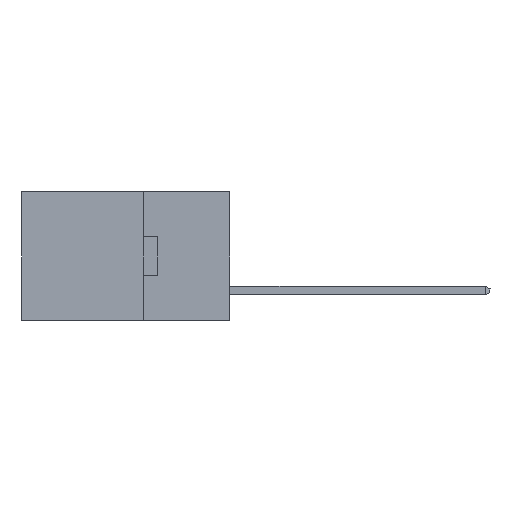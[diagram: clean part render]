
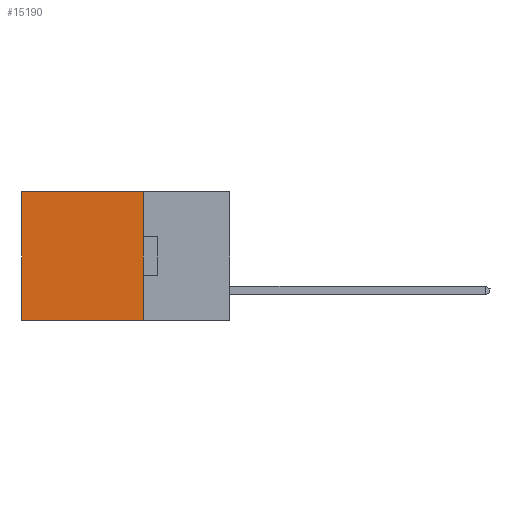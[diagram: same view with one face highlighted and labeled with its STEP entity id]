
A CAD part, left-side view. The second image highlights one B-rep face of the part: STEP entity #15190.
In plain terms, the highlighted planar face has unit normal (-1, 0, 0).
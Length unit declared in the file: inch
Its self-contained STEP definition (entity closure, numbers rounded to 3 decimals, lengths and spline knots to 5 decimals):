
#1977 = DIRECTION ( 'NONE',  ( 0., 1., 0. ) ) ;
#2540 = CARTESIAN_POINT ( 'NONE',  ( 0.2615, 0.6, -0.37 ) ) ;
#4288 = EDGE_LOOP ( 'NONE', ( #26540, #19473, #7708, #11205 ) ) ;
#7142 = VERTEX_POINT ( 'NONE', #14730 ) ;
#7708 = ORIENTED_EDGE ( 'NONE', *, *, #24120, .F. ) ;
#8115 = CARTESIAN_POINT ( 'NONE',  ( 0.2615, 0.25, -0.37 ) ) ;
#9136 = LINE ( 'NONE', #2540, #27112 ) ;
#9703 = DIRECTION ( 'NONE',  ( 0., 0., -1. ) ) ;
#11191 = VECTOR ( 'NONE', #24439, 39.37008 ) ;
#11205 = ORIENTED_EDGE ( 'NONE', *, *, #12242, .T. ) ;
#12172 = CARTESIAN_POINT ( 'NONE',  ( 0.2615, 0.25, 0. ) ) ;
#12242 = EDGE_CURVE ( 'NONE', #23742, #7142, #24299, .T. ) ;
#13136 = CARTESIAN_POINT ( 'NONE',  ( 0.2615, 0.6, -0.37 ) ) ;
#14111 = EDGE_CURVE ( 'NONE', #15442, #15092, #14887, .T. ) ;
#14730 = CARTESIAN_POINT ( 'NONE',  ( 0.2615, 0.6, 0. ) ) ;
#14887 = LINE ( 'NONE', #27142, #22099 ) ;
#15020 = CARTESIAN_POINT ( 'NONE',  ( 0.2615, 0.25, -0.37 ) ) ;
#15092 = VERTEX_POINT ( 'NONE', #13136 ) ;
#15190 = ADVANCED_FACE ( 'NONE', ( #18088 ), #22358, .F. ) ;
#15442 = VERTEX_POINT ( 'NONE', #15020 ) ;
#16292 = CARTESIAN_POINT ( 'NONE',  ( 0.2615, 0.25, -0.37 ) ) ;
#18001 = VECTOR ( 'NONE', #23085, 39.37008 ) ;
#18088 = FACE_OUTER_BOUND ( 'NONE', #4288, .T. ) ;
#18872 = EDGE_CURVE ( 'NONE', #7142, #15092, #9136, .T. ) ;
#19466 = DIRECTION ( 'NONE',  ( 0., 0., -1. ) ) ;
#19473 = ORIENTED_EDGE ( 'NONE', *, *, #14111, .F. ) ;
#20189 = CARTESIAN_POINT ( 'NONE',  ( 0.2615, 0.25, 0. ) ) ;
#22099 = VECTOR ( 'NONE', #1977, 39.37008 ) ;
#22358 = PLANE ( 'NONE',  #26960 ) ;
#22691 = LINE ( 'NONE', #8115, #18001 ) ;
#23085 = DIRECTION ( 'NONE',  ( 0., 0., -1. ) ) ;
#23742 = VERTEX_POINT ( 'NONE', #12172 ) ;
#24120 = EDGE_CURVE ( 'NONE', #23742, #15442, #22691, .T. ) ;
#24299 = LINE ( 'NONE', #20189, #11191 ) ;
#24439 = DIRECTION ( 'NONE',  ( 0., 1., 0. ) ) ;
#26540 = ORIENTED_EDGE ( 'NONE', *, *, #18872, .T. ) ;
#26960 = AXIS2_PLACEMENT_3D ( 'NONE', #16292, #27020, #9703 ) ;
#27020 = DIRECTION ( 'NONE',  ( 1., 0., 0. ) ) ;
#27112 = VECTOR ( 'NONE', #19466, 39.37008 ) ;
#27142 = CARTESIAN_POINT ( 'NONE',  ( 0.2615, 0.25, -0.37 ) ) ;
